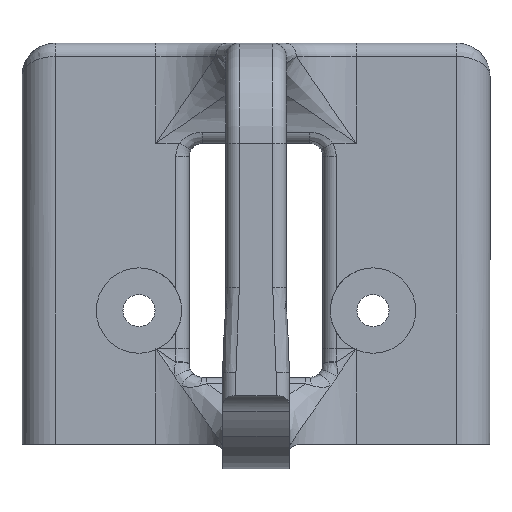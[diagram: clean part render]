
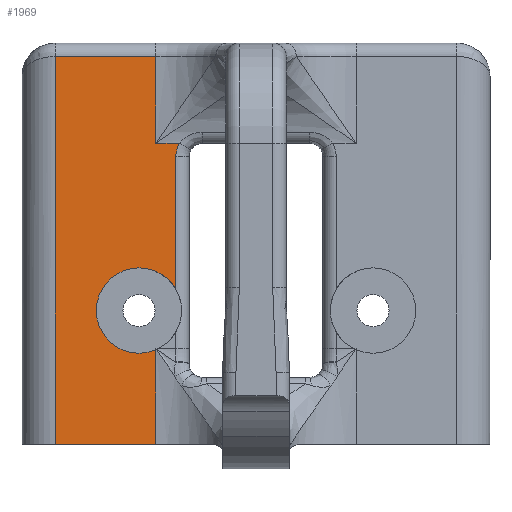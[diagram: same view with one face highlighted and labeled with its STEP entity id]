
A CAD part, front view. The second image highlights one B-rep face of the part: STEP entity #1969.
In plain terms, the highlighted planar face has unit normal (0, -1, 0).
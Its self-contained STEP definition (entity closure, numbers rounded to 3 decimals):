
#98 = VERTEX_POINT ( 'NONE', #3465 ) ;
#199 = FACE_OUTER_BOUND ( 'NONE', #1178, .T. ) ;
#218 = VECTOR ( 'NONE', #2599, 1000. ) ;
#336 = EDGE_CURVE ( 'NONE', #1185, #1334, #3055, .T. ) ;
#355 = CARTESIAN_POINT ( 'NONE',  ( -12.5, 7.5, 0. ) ) ;
#370 = ORIENTED_EDGE ( 'NONE', *, *, #1011, .T. ) ;
#397 = AXIS2_PLACEMENT_3D ( 'NONE', #3548, #1218, #4188 ) ;
#513 = ORIENTED_EDGE ( 'NONE', *, *, #1096, .T. ) ;
#603 = CARTESIAN_POINT ( 'NONE',  ( 5., 7.5, 0. ) ) ;
#607 = EDGE_CURVE ( 'NONE', #98, #2251, #2617, .T. ) ;
#619 = LINE ( 'NONE', #355, #631 ) ;
#621 = CARTESIAN_POINT ( 'NONE',  ( -6.25, 7.5, -5. ) ) ;
#624 = VERTEX_POINT ( 'NONE', #3726 ) ;
#631 = VECTOR ( 'NONE', #2623, 1000. ) ;
#683 = VERTEX_POINT ( 'NONE', #3561 ) ;
#698 = PLANE ( 'NONE',  #3970 ) ;
#763 = AXIS2_PLACEMENT_3D ( 'NONE', #2181, #2168, #2148 ) ;
#806 = EDGE_CURVE ( 'NONE', #624, #2411, #2277, .T. ) ;
#875 = VERTEX_POINT ( 'NONE', #2911 ) ;
#930 = DIRECTION ( 'NONE',  ( 0., 0., -1. ) ) ;
#944 = DIRECTION ( 'NONE',  ( 0., 0., -1. ) ) ;
#1011 = EDGE_CURVE ( 'NONE', #683, #1863, #1959, .T. ) ;
#1017 = ORIENTED_EDGE ( 'NONE', *, *, #607, .T. ) ;
#1055 = AXIS2_PLACEMENT_3D ( 'NONE', #621, #2913, #944 ) ;
#1070 = ORIENTED_EDGE ( 'NONE', *, *, #2236, .F. ) ;
#1096 = EDGE_CURVE ( 'NONE', #2251, #683, #1892, .T. ) ;
#1145 = CARTESIAN_POINT ( 'NONE',  ( -12.5, 7.5, 14. ) ) ;
#1178 = EDGE_LOOP ( 'NONE', ( #1017, #513, #370, #2763, #2176, #3512, #1629, #3783, #1070, #3229, #1492 ) ) ;
#1185 = VERTEX_POINT ( 'NONE', #2035 ) ;
#1218 = DIRECTION ( 'NONE',  ( 0., -1., 0. ) ) ;
#1317 = VERTEX_POINT ( 'NONE', #1516 ) ;
#1334 = VERTEX_POINT ( 'NONE', #1407 ) ;
#1380 = CIRCLE ( 'NONE', #1055, 3.19 ) ;
#1407 = CARTESIAN_POINT ( 'NONE',  ( -5., 7.5, -7.935 ) ) ;
#1492 = ORIENTED_EDGE ( 'NONE', *, *, #2007, .F. ) ;
#1516 = CARTESIAN_POINT ( 'NONE',  ( -6.25, 7.5, -8.19 ) ) ;
#1629 = ORIENTED_EDGE ( 'NONE', *, *, #2812, .F. ) ;
#1663 = EDGE_CURVE ( 'NONE', #2411, #3424, #619, .T. ) ;
#1863 = VERTEX_POINT ( 'NONE', #3867 ) ;
#1892 = CIRCLE ( 'NONE', #763, 2. ) ;
#1909 = DIRECTION ( 'NONE',  ( -1., 0., 0. ) ) ;
#1953 = VECTOR ( 'NONE', #1909, 1000. ) ;
#1959 = LINE ( 'NONE', #2520, #1953 ) ;
#1969 = ADVANCED_FACE ( 'NONE', ( #199 ), #698, .T. ) ;
#2007 = EDGE_CURVE ( 'NONE', #98, #875, #1380, .T. ) ;
#2035 = CARTESIAN_POINT ( 'NONE',  ( -5., 7.5, -15. ) ) ;
#2148 = DIRECTION ( 'NONE',  ( 0., 0., -1. ) ) ;
#2168 = DIRECTION ( 'NONE',  ( 0., 1., 0. ) ) ;
#2176 = ORIENTED_EDGE ( 'NONE', *, *, #806, .T. ) ;
#2181 = CARTESIAN_POINT ( 'NONE',  ( -1.5, 7.5, 6.5 ) ) ;
#2236 = EDGE_CURVE ( 'NONE', #1317, #1334, #3104, .T. ) ;
#2251 = VERTEX_POINT ( 'NONE', #2998 ) ;
#2277 = LINE ( 'NONE', #3169, #2372 ) ;
#2372 = VECTOR ( 'NONE', #3124, 1000. ) ;
#2411 = VERTEX_POINT ( 'NONE', #1145 ) ;
#2520 = CARTESIAN_POINT ( 'NONE',  ( 5., 7.5, 7.5 ) ) ;
#2553 = EDGE_CURVE ( 'NONE', #1863, #624, #2930, .T. ) ;
#2559 = VECTOR ( 'NONE', #3798, 1000. ) ;
#2592 = CARTESIAN_POINT ( 'NONE',  ( -15., 7.5, -15. ) ) ;
#2599 = DIRECTION ( 'NONE',  ( -1., 0., 0. ) ) ;
#2617 = LINE ( 'NONE', #3836, #2559 ) ;
#2623 = DIRECTION ( 'NONE',  ( 0., 0., -1. ) ) ;
#2763 = ORIENTED_EDGE ( 'NONE', *, *, #2553, .T. ) ;
#2812 = EDGE_CURVE ( 'NONE', #1185, #3424, #3698, .T. ) ;
#2903 = DIRECTION ( 'NONE',  ( 0., -1., 0. ) ) ;
#2911 = CARTESIAN_POINT ( 'NONE',  ( -6.25, 7.5, -1.81 ) ) ;
#2913 = DIRECTION ( 'NONE',  ( 0., -1., 0. ) ) ;
#2930 = LINE ( 'NONE', #3995, #3160 ) ;
#2943 = VECTOR ( 'NONE', #4101, 1000. ) ;
#2998 = CARTESIAN_POINT ( 'NONE',  ( -3.5, 7.5, 6.5 ) ) ;
#3042 = DIRECTION ( 'NONE',  ( 0., 0., -1. ) ) ;
#3055 = LINE ( 'NONE', #4088, #2943 ) ;
#3060 = DIRECTION ( 'NONE',  ( 0., -1., 0. ) ) ;
#3066 = CARTESIAN_POINT ( 'NONE',  ( -6.25, 7.5, -5. ) ) ;
#3104 = CIRCLE ( 'NONE', #3649, 3.19 ) ;
#3124 = DIRECTION ( 'NONE',  ( -1., 0., 0. ) ) ;
#3160 = VECTOR ( 'NONE', #4069, 1000. ) ;
#3169 = CARTESIAN_POINT ( 'NONE',  ( 5., 7.5, 14. ) ) ;
#3229 = ORIENTED_EDGE ( 'NONE', *, *, #4028, .F. ) ;
#3424 = VERTEX_POINT ( 'NONE', #3823 ) ;
#3465 = CARTESIAN_POINT ( 'NONE',  ( -3.5, 7.5, -3.383 ) ) ;
#3512 = ORIENTED_EDGE ( 'NONE', *, *, #1663, .T. ) ;
#3548 = CARTESIAN_POINT ( 'NONE',  ( -6.25, 7.5, -5. ) ) ;
#3561 = CARTESIAN_POINT ( 'NONE',  ( -3.232, 7.5, 7.5 ) ) ;
#3649 = AXIS2_PLACEMENT_3D ( 'NONE', #3066, #3060, #3042 ) ;
#3698 = LINE ( 'NONE', #2592, #218 ) ;
#3726 = CARTESIAN_POINT ( 'NONE',  ( -5., 7.5, 14. ) ) ;
#3783 = ORIENTED_EDGE ( 'NONE', *, *, #336, .T. ) ;
#3798 = DIRECTION ( 'NONE',  ( 0., 0., 1. ) ) ;
#3823 = CARTESIAN_POINT ( 'NONE',  ( -12.5, 7.5, -15. ) ) ;
#3836 = CARTESIAN_POINT ( 'NONE',  ( -3.5, 7.5, 6.5 ) ) ;
#3867 = CARTESIAN_POINT ( 'NONE',  ( -5., 7.5, 7.5 ) ) ;
#3970 = AXIS2_PLACEMENT_3D ( 'NONE', #603, #2903, #930 ) ;
#3995 = CARTESIAN_POINT ( 'NONE',  ( -5., 7.5, 0. ) ) ;
#4023 = CIRCLE ( 'NONE', #397, 3.19 ) ;
#4028 = EDGE_CURVE ( 'NONE', #875, #1317, #4023, .T. ) ;
#4069 = DIRECTION ( 'NONE',  ( 0., 0., 1. ) ) ;
#4088 = CARTESIAN_POINT ( 'NONE',  ( -5., 7.5, 0. ) ) ;
#4101 = DIRECTION ( 'NONE',  ( 0., 0., 1. ) ) ;
#4188 = DIRECTION ( 'NONE',  ( 0., 0., -1. ) ) ;
